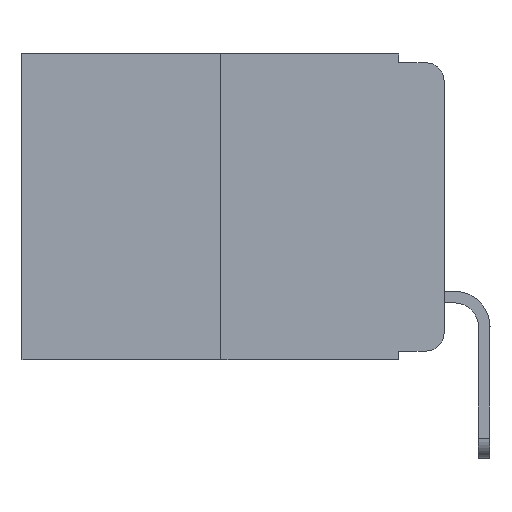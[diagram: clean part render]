
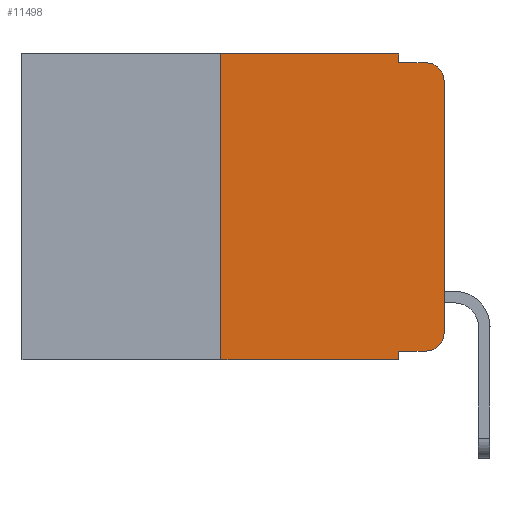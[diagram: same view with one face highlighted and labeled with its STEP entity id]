
A CAD part, left-side view. The second image highlights one B-rep face of the part: STEP entity #11498.
In plain terms, the highlighted planar face has unit normal (-1, 0, 0).
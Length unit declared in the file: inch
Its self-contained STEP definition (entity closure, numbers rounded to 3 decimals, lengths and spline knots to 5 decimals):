
#334 = DIRECTION ( 'NONE',  ( -1., 0., 0. ) ) ;
#358 = CARTESIAN_POINT ( 'NONE',  ( 0., 0.02, -0.333 ) ) ;
#419 = DIRECTION ( 'NONE',  ( 0., -1., 0. ) ) ;
#423 = CARTESIAN_POINT ( 'NONE',  ( 0., 0.25, 0. ) ) ;
#601 = LINE ( 'NONE', #14418, #17974 ) ;
#812 = VERTEX_POINT ( 'NONE', #16629 ) ;
#822 = LINE ( 'NONE', #6468, #14595 ) ;
#963 = VECTOR ( 'NONE', #12755, 39.37008 ) ;
#1228 = DIRECTION ( 'NONE',  ( 1., 0., 0. ) ) ;
#2740 = AXIS2_PLACEMENT_3D ( 'NONE', #12941, #334, #8703 ) ;
#2926 = ORIENTED_EDGE ( 'NONE', *, *, #16575, .F. ) ;
#2972 = CARTESIAN_POINT ( 'NONE',  ( 0., 0.02, -0.313 ) ) ;
#3125 = VECTOR ( 'NONE', #8894, 39.37008 ) ;
#3174 = VERTEX_POINT ( 'NONE', #16205 ) ;
#3340 = CARTESIAN_POINT ( 'NONE',  ( 0., 0.25, -0.343 ) ) ;
#3697 = ORIENTED_EDGE ( 'NONE', *, *, #16054, .T. ) ;
#3814 = PLANE ( 'NONE',  #11835 ) ;
#4093 = CARTESIAN_POINT ( 'NONE',  ( 0., 0.051, -0.343 ) ) ;
#4668 = AXIS2_PLACEMENT_3D ( 'NONE', #2972, #12995, #11531 ) ;
#4841 = DIRECTION ( 'NONE',  ( 0., -1., 0. ) ) ;
#4949 = CARTESIAN_POINT ( 'NONE',  ( 0., 0., 0. ) ) ;
#5388 = DIRECTION ( 'NONE',  ( 0., 0., -1. ) ) ;
#5926 = CARTESIAN_POINT ( 'NONE',  ( 0., 0.051, -0.333 ) ) ;
#6153 = LINE ( 'NONE', #10185, #12109 ) ;
#6339 = LINE ( 'NONE', #4949, #3125 ) ;
#6468 = CARTESIAN_POINT ( 'NONE',  ( 0., 0.051, 0. ) ) ;
#6476 = LINE ( 'NONE', #11042, #14618 ) ;
#6605 = EDGE_CURVE ( 'NONE', #13913, #15358, #11382, .T. ) ;
#6668 = EDGE_CURVE ( 'NONE', #16935, #812, #14513, .T. ) ;
#6944 = ORIENTED_EDGE ( 'NONE', *, *, #17152, .F. ) ;
#7243 = EDGE_CURVE ( 'NONE', #15723, #3174, #822, .T. ) ;
#7506 = VERTEX_POINT ( 'NONE', #358 ) ;
#8060 = EDGE_CURVE ( 'NONE', #3174, #812, #601, .T. ) ;
#8306 = DIRECTION ( 'NONE',  ( 0., -1., 0. ) ) ;
#8494 = CARTESIAN_POINT ( 'NONE',  ( 0., 0.473, 0. ) ) ;
#8703 = DIRECTION ( 'NONE',  ( 0., 0., -1. ) ) ;
#8760 = CARTESIAN_POINT ( 'NONE',  ( 0., 0., -0.03 ) ) ;
#8894 = DIRECTION ( 'NONE',  ( 0., 0., 1. ) ) ;
#9250 = ORIENTED_EDGE ( 'NONE', *, *, #6605, .F. ) ;
#9534 = CARTESIAN_POINT ( 'NONE',  ( 0., 0.473, -0.343 ) ) ;
#9565 = CARTESIAN_POINT ( 'NONE',  ( 0., 0., -0.313 ) ) ;
#9849 = EDGE_CURVE ( 'NONE', #13913, #11554, #16548, .T. ) ;
#9882 = EDGE_LOOP ( 'NONE', ( #3697, #12465, #12667, #16301, #2926, #9250, #10851, #6944, #17753, #9974 ) ) ;
#9974 = ORIENTED_EDGE ( 'NONE', *, *, #18089, .T. ) ;
#10185 = CARTESIAN_POINT ( 'NONE',  ( 0., 0.051, -0.333 ) ) ;
#10851 = ORIENTED_EDGE ( 'NONE', *, *, #9849, .T. ) ;
#10933 = CARTESIAN_POINT ( 'NONE',  ( 0., 0.051, 0. ) ) ;
#11042 = CARTESIAN_POINT ( 'NONE',  ( 0., 0.051, 0. ) ) ;
#11194 = EDGE_CURVE ( 'NONE', #12113, #7506, #6153, .T. ) ;
#11382 = LINE ( 'NONE', #423, #963 ) ;
#11498 = ADVANCED_FACE ( 'NONE', ( #15145 ), #3814, .F. ) ;
#11531 = DIRECTION ( 'NONE',  ( 0., 0., -1. ) ) ;
#11554 = VERTEX_POINT ( 'NONE', #4093 ) ;
#11835 = AXIS2_PLACEMENT_3D ( 'NONE', #17985, #1228, #5388 ) ;
#12109 = VECTOR ( 'NONE', #14324, 39.37008 ) ;
#12113 = VERTEX_POINT ( 'NONE', #5926 ) ;
#12335 = CARTESIAN_POINT ( 'NONE',  ( 0., 0.25, 0. ) ) ;
#12391 = VERTEX_POINT ( 'NONE', #9565 ) ;
#12465 = ORIENTED_EDGE ( 'NONE', *, *, #6668, .T. ) ;
#12667 = ORIENTED_EDGE ( 'NONE', *, *, #8060, .F. ) ;
#12755 = DIRECTION ( 'NONE',  ( 0., 0., 1. ) ) ;
#12941 = CARTESIAN_POINT ( 'NONE',  ( 0., 0.02, -0.03 ) ) ;
#12995 = DIRECTION ( 'NONE',  ( -1., 0., 0. ) ) ;
#13757 = CIRCLE ( 'NONE', #4668, 0.02 ) ;
#13913 = VERTEX_POINT ( 'NONE', #3340 ) ;
#14324 = DIRECTION ( 'NONE',  ( 0., -1., 0. ) ) ;
#14418 = CARTESIAN_POINT ( 'NONE',  ( 0., 0.051, -0.01 ) ) ;
#14513 = CIRCLE ( 'NONE', #2740, 0.02 ) ;
#14595 = VECTOR ( 'NONE', #15107, 39.37008 ) ;
#14618 = VECTOR ( 'NONE', #16504, 39.37008 ) ;
#15107 = DIRECTION ( 'NONE',  ( 0., 0., -1. ) ) ;
#15145 = FACE_OUTER_BOUND ( 'NONE', #9882, .T. ) ;
#15358 = VERTEX_POINT ( 'NONE', #12335 ) ;
#15723 = VERTEX_POINT ( 'NONE', #10933 ) ;
#16054 = EDGE_CURVE ( 'NONE', #12391, #16935, #6339, .T. ) ;
#16205 = CARTESIAN_POINT ( 'NONE',  ( 0., 0.051, -0.01 ) ) ;
#16301 = ORIENTED_EDGE ( 'NONE', *, *, #7243, .F. ) ;
#16389 = VECTOR ( 'NONE', #8306, 39.37008 ) ;
#16504 = DIRECTION ( 'NONE',  ( 0., 0., -1. ) ) ;
#16548 = LINE ( 'NONE', #9534, #17695 ) ;
#16575 = EDGE_CURVE ( 'NONE', #15358, #15723, #16802, .T. ) ;
#16629 = CARTESIAN_POINT ( 'NONE',  ( 0., 0.02, -0.01 ) ) ;
#16802 = LINE ( 'NONE', #8494, #16389 ) ;
#16935 = VERTEX_POINT ( 'NONE', #8760 ) ;
#17152 = EDGE_CURVE ( 'NONE', #12113, #11554, #6476, .T. ) ;
#17695 = VECTOR ( 'NONE', #419, 39.37008 ) ;
#17753 = ORIENTED_EDGE ( 'NONE', *, *, #11194, .T. ) ;
#17974 = VECTOR ( 'NONE', #4841, 39.37008 ) ;
#17985 = CARTESIAN_POINT ( 'NONE',  ( 0., 0.473, 0. ) ) ;
#18089 = EDGE_CURVE ( 'NONE', #7506, #12391, #13757, .T. ) ;
